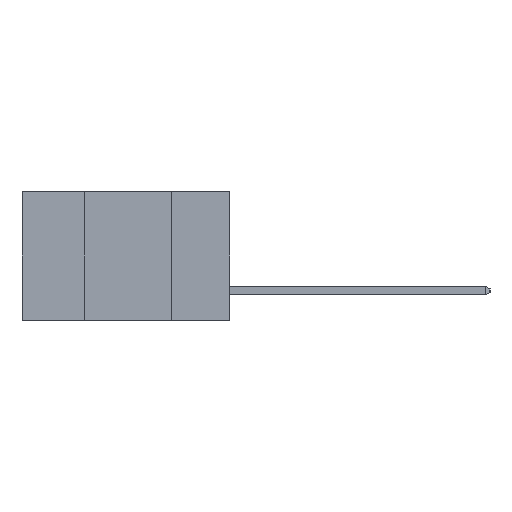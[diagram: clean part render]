
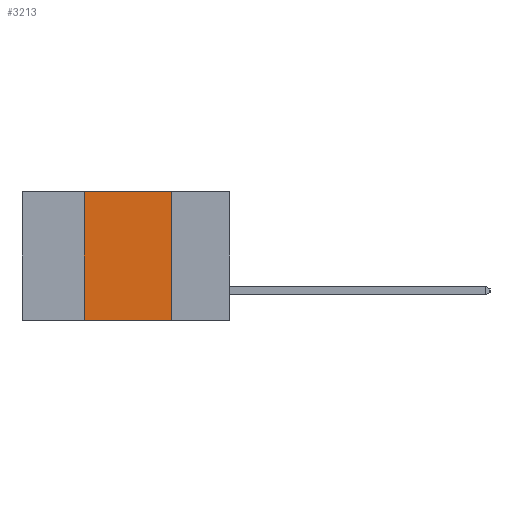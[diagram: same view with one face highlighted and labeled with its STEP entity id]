
A CAD part, left-side view. The second image highlights one B-rep face of the part: STEP entity #3213.
In plain terms, the highlighted planar face has unit normal (-1, 0, 0).
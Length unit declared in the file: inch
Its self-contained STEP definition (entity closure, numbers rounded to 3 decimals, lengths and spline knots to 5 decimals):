
#251 = LINE ( 'NONE', #11184, #8652 ) ;
#397 = VERTEX_POINT ( 'NONE', #6663 ) ;
#429 = ORIENTED_EDGE ( 'NONE', *, *, #4768, .F. ) ;
#519 = PLANE ( 'NONE',  #4929 ) ;
#798 = LINE ( 'NONE', #11221, #8169 ) ;
#1295 = ORIENTED_EDGE ( 'NONE', *, *, #6230, .T. ) ;
#1430 = LINE ( 'NONE', #3398, #6691 ) ;
#1866 = CARTESIAN_POINT ( 'NONE',  ( 0., 0.42, -0.37 ) ) ;
#2021 = EDGE_LOOP ( 'NONE', ( #4453, #429, #5122, #1295 ) ) ;
#2943 = EDGE_CURVE ( 'NONE', #6119, #397, #1430, .T. ) ;
#3213 = ADVANCED_FACE ( 'NONE', ( #11583 ), #519, .F. ) ;
#3398 = CARTESIAN_POINT ( 'NONE',  ( 0., 0.17, -0.37 ) ) ;
#4110 = DIRECTION ( 'NONE',  ( 0., -1., 0. ) ) ;
#4380 = VECTOR ( 'NONE', #10470, 39.37008 ) ;
#4453 = ORIENTED_EDGE ( 'NONE', *, *, #2943, .F. ) ;
#4768 = EDGE_CURVE ( 'NONE', #6199, #6119, #7104, .T. ) ;
#4929 = AXIS2_PLACEMENT_3D ( 'NONE', #8894, #12320, #12555 ) ;
#4958 = CARTESIAN_POINT ( 'NONE',  ( 0., 0.17, 0. ) ) ;
#5122 = ORIENTED_EDGE ( 'NONE', *, *, #7508, .F. ) ;
#6119 = VERTEX_POINT ( 'NONE', #4958 ) ;
#6199 = VERTEX_POINT ( 'NONE', #11175 ) ;
#6230 = EDGE_CURVE ( 'NONE', #6834, #397, #798, .T. ) ;
#6663 = CARTESIAN_POINT ( 'NONE',  ( 0., 0.17, -0.37 ) ) ;
#6691 = VECTOR ( 'NONE', #7577, 39.37008 ) ;
#6834 = VERTEX_POINT ( 'NONE', #1866 ) ;
#7104 = LINE ( 'NONE', #8434, #4380 ) ;
#7508 = EDGE_CURVE ( 'NONE', #6834, #6199, #251, .T. ) ;
#7577 = DIRECTION ( 'NONE',  ( 0., 0., -1. ) ) ;
#8142 = DIRECTION ( 'NONE',  ( 0., 0., 1. ) ) ;
#8169 = VECTOR ( 'NONE', #4110, 39.37008 ) ;
#8434 = CARTESIAN_POINT ( 'NONE',  ( 0., 0.6, 0. ) ) ;
#8652 = VECTOR ( 'NONE', #8142, 39.37008 ) ;
#8894 = CARTESIAN_POINT ( 'NONE',  ( 0., 0.6, 0. ) ) ;
#10470 = DIRECTION ( 'NONE',  ( 0., -1., 0. ) ) ;
#11175 = CARTESIAN_POINT ( 'NONE',  ( 0., 0.42, 0. ) ) ;
#11184 = CARTESIAN_POINT ( 'NONE',  ( 0., 0.42, -0.37 ) ) ;
#11221 = CARTESIAN_POINT ( 'NONE',  ( 0., 0.6, -0.37 ) ) ;
#11583 = FACE_OUTER_BOUND ( 'NONE', #2021, .T. ) ;
#12320 = DIRECTION ( 'NONE',  ( 1., 0., 0. ) ) ;
#12555 = DIRECTION ( 'NONE',  ( 0., 0., -1. ) ) ;
